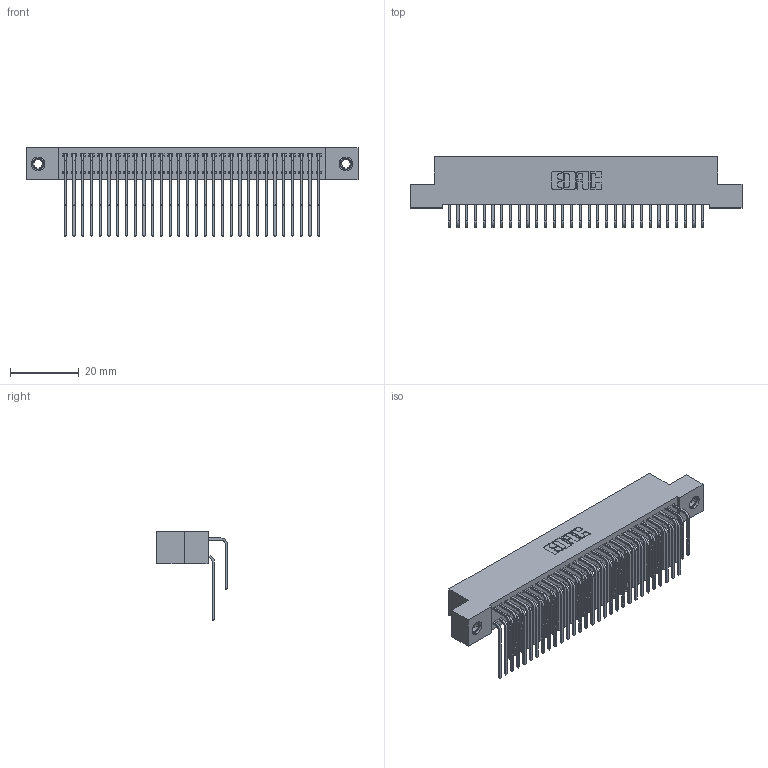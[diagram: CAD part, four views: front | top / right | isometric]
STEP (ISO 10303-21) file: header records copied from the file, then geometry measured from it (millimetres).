
FILE_DESCRIPTION (( 'STEP AP203' ), '1' );
FILE_NAME ('342-060-559-207.STEP', '2019-10-03T13:37:42', ( '' ), ( '' ), 'SwSTEP 2.0', 'SolidWorks 2016', '' );
FILE_SCHEMA (( 'CONFIG_CONTROL_DESIGN' ));
Length unit declared in the file: inch
Products named in the file (5): 342 Part_TI; 345-292-001_558 559 Tail - 1; 345-292-001_559 Tail - 2; 345-250-001_345-250-005-103; 342-060-559-207
Assembly tree (63 placements, depth 2):
  342-060-559-207
    342 Part_TI
    345-292-001_558 559 Tail - 1  x30
    345-292-001_559 Tail - 2  x30
    345-250-001_345-250-005-103  x2
Bounding box: 96.52 x 20.64 x 25.78 mm (x, y, z)
Volume: 8948.9 mm3; surface area: 15862.5 mm2
Topology: 63 solids, 63 shells, 3410 faces, 10095 edges, 6642 vertices
Faces by surface type: plane 2378, cylinder 1016, cone 12, torus 4
Entity records: 23690 total; most frequent: CARTESIAN_POINT 3972, ORIENTED_EDGE 3850, DIRECTION 3427, EDGE_CURVE 1925, VECTOR 1737, LINE 1737, VERTEX_POINT 1276, AXIS2_PLACEMENT_3D 845
